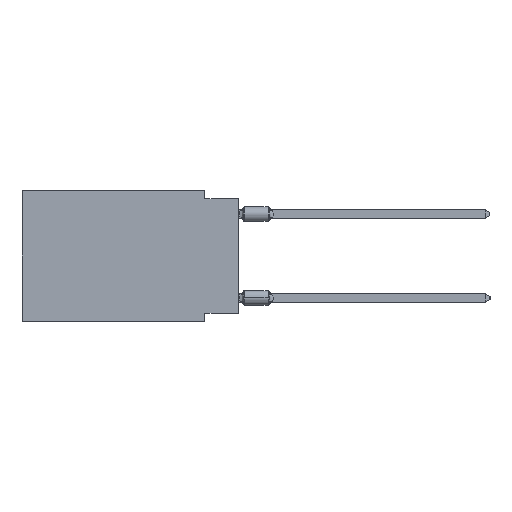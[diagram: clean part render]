
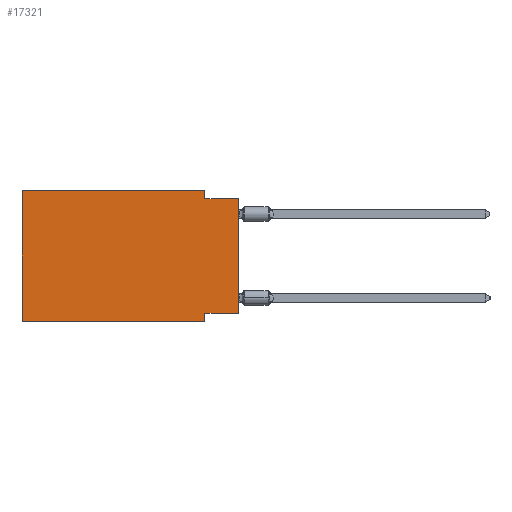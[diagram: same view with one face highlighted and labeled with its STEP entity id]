
A CAD part, left-side view. The second image highlights one B-rep face of the part: STEP entity #17321.
In plain terms, the highlighted planar face has unit normal (-1, 0, 0).
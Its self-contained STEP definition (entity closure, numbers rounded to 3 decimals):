
#149 = CARTESIAN_POINT ( 'NONE',  ( 0., 2.54, 0. ) ) ;
#837 = CARTESIAN_POINT ( 'NONE',  ( 0., 2.54, 0. ) ) ;
#1527 = CARTESIAN_POINT ( 'NONE',  ( 0., 16.383, 0. ) ) ;
#1793 = CARTESIAN_POINT ( 'NONE',  ( 0., 2.54, -0.635 ) ) ;
#2073 = VERTEX_POINT ( 'NONE', #837 ) ;
#3268 = LINE ( 'NONE', #149, #38466 ) ;
#3596 = VERTEX_POINT ( 'NONE', #26732 ) ;
#3736 = AXIS2_PLACEMENT_3D ( 'NONE', #1527, #10068, #39281 ) ;
#3779 = ORIENTED_EDGE ( 'NONE', *, *, #29963, .F. ) ;
#4367 = VERTEX_POINT ( 'NONE', #19867 ) ;
#5187 = DIRECTION ( 'NONE',  ( 0., 0., -1. ) ) ;
#6611 = LINE ( 'NONE', #19276, #38730 ) ;
#8558 = ORIENTED_EDGE ( 'NONE', *, *, #22094, .F. ) ;
#8716 = EDGE_CURVE ( 'NONE', #4367, #34364, #22409, .T. ) ;
#8807 = CARTESIAN_POINT ( 'NONE',  ( 0., 0., -0.635 ) ) ;
#8964 = CARTESIAN_POINT ( 'NONE',  ( 0., 2.54, -9.271 ) ) ;
#9972 = CARTESIAN_POINT ( 'NONE',  ( 0., 16.383, 0. ) ) ;
#10068 = DIRECTION ( 'NONE',  ( 1., 0., 0. ) ) ;
#11194 = EDGE_CURVE ( 'NONE', #31139, #20004, #24979, .T. ) ;
#11436 = LINE ( 'NONE', #14752, #36720 ) ;
#12396 = CARTESIAN_POINT ( 'NONE',  ( 0., 0., -0.635 ) ) ;
#12822 = DIRECTION ( 'NONE',  ( 0., 0., -1. ) ) ;
#12856 = CARTESIAN_POINT ( 'NONE',  ( 0., 16.383, 0. ) ) ;
#13012 = CARTESIAN_POINT ( 'NONE',  ( 0., 0., -9.271 ) ) ;
#14555 = VERTEX_POINT ( 'NONE', #1793 ) ;
#14752 = CARTESIAN_POINT ( 'NONE',  ( 0., 2.54, -9.906 ) ) ;
#15304 = LINE ( 'NONE', #12396, #16447 ) ;
#15656 = CARTESIAN_POINT ( 'NONE',  ( 0., 16.383, -9.906 ) ) ;
#15750 = DIRECTION ( 'NONE',  ( 0., -1., 0. ) ) ;
#16447 = VECTOR ( 'NONE', #18206, 1000. ) ;
#17081 = EDGE_CURVE ( 'NONE', #4367, #3596, #34336, .T. ) ;
#17321 = ADVANCED_FACE ( 'NONE', ( #36167 ), #19802, .F. ) ;
#18206 = DIRECTION ( 'NONE',  ( 0., -1., 0. ) ) ;
#18863 = VECTOR ( 'NONE', #25665, 1000. ) ;
#18997 = ORIENTED_EDGE ( 'NONE', *, *, #22261, .F. ) ;
#19262 = VERTEX_POINT ( 'NONE', #8964 ) ;
#19276 = CARTESIAN_POINT ( 'NONE',  ( 0., 16.383, 0. ) ) ;
#19802 = PLANE ( 'NONE',  #3736 ) ;
#19867 = CARTESIAN_POINT ( 'NONE',  ( 0., 16.383, -9.906 ) ) ;
#20004 = VERTEX_POINT ( 'NONE', #8807 ) ;
#20833 = CARTESIAN_POINT ( 'NONE',  ( 0., 0., 0. ) ) ;
#21252 = DIRECTION ( 'NONE',  ( 0., 0., 1. ) ) ;
#22094 = EDGE_CURVE ( 'NONE', #19262, #3596, #11436, .T. ) ;
#22261 = EDGE_CURVE ( 'NONE', #34364, #2073, #6611, .T. ) ;
#22409 = LINE ( 'NONE', #9972, #39820 ) ;
#22611 = DIRECTION ( 'NONE',  ( 0., 0., 1. ) ) ;
#22735 = EDGE_CURVE ( 'NONE', #31139, #19262, #27046, .T. ) ;
#24271 = ORIENTED_EDGE ( 'NONE', *, *, #17081, .T. ) ;
#24979 = LINE ( 'NONE', #20833, #31991 ) ;
#25618 = EDGE_LOOP ( 'NONE', ( #29430, #29954, #3779, #18997, #37333, #24271, #8558, #27307 ) ) ;
#25665 = DIRECTION ( 'NONE',  ( 0., 1., 0. ) ) ;
#26732 = CARTESIAN_POINT ( 'NONE',  ( 0., 2.54, -9.906 ) ) ;
#26852 = EDGE_CURVE ( 'NONE', #14555, #20004, #15304, .T. ) ;
#27046 = LINE ( 'NONE', #13012, #18863 ) ;
#27307 = ORIENTED_EDGE ( 'NONE', *, *, #22735, .F. ) ;
#29430 = ORIENTED_EDGE ( 'NONE', *, *, #11194, .T. ) ;
#29954 = ORIENTED_EDGE ( 'NONE', *, *, #26852, .F. ) ;
#29963 = EDGE_CURVE ( 'NONE', #2073, #14555, #3268, .T. ) ;
#31139 = VERTEX_POINT ( 'NONE', #35881 ) ;
#31991 = VECTOR ( 'NONE', #21252, 1000. ) ;
#34336 = LINE ( 'NONE', #15656, #36891 ) ;
#34364 = VERTEX_POINT ( 'NONE', #12856 ) ;
#35881 = CARTESIAN_POINT ( 'NONE',  ( 0., 0., -9.271 ) ) ;
#36167 = FACE_OUTER_BOUND ( 'NONE', #25618, .T. ) ;
#36720 = VECTOR ( 'NONE', #5187, 1000. ) ;
#36891 = VECTOR ( 'NONE', #38054, 1000. ) ;
#37333 = ORIENTED_EDGE ( 'NONE', *, *, #8716, .F. ) ;
#38054 = DIRECTION ( 'NONE',  ( 0., -1., 0. ) ) ;
#38466 = VECTOR ( 'NONE', #12822, 1000. ) ;
#38730 = VECTOR ( 'NONE', #15750, 1000. ) ;
#39281 = DIRECTION ( 'NONE',  ( 0., 0., -1. ) ) ;
#39820 = VECTOR ( 'NONE', #22611, 1000. ) ;
